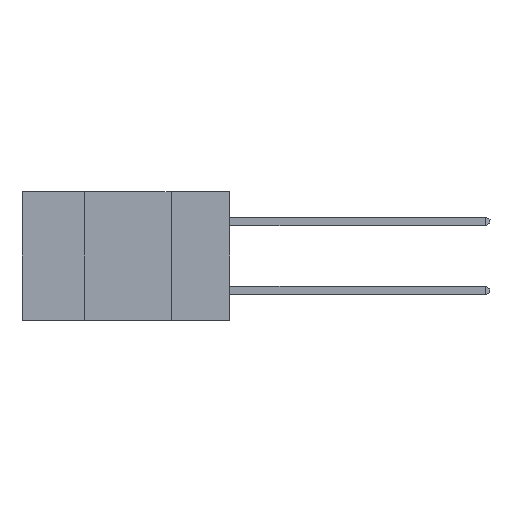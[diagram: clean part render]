
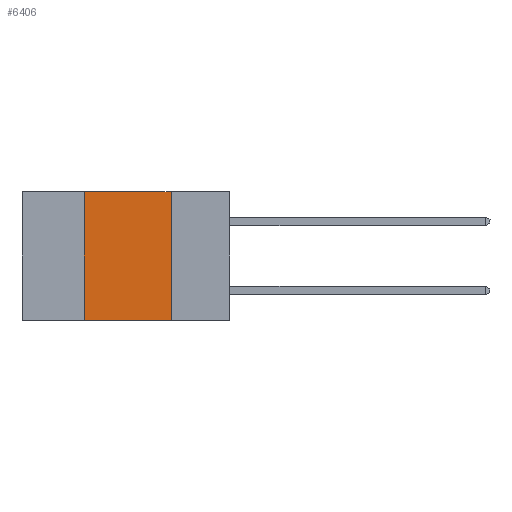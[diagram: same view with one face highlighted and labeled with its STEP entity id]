
A CAD part, left-side view. The second image highlights one B-rep face of the part: STEP entity #6406.
In plain terms, the highlighted planar face has unit normal (-1, 0, 0).
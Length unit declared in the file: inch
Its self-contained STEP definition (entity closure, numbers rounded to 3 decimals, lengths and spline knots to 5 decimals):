
#94 = FACE_OUTER_BOUND ( 'NONE', #4896, .T. ) ;
#142 = VERTEX_POINT ( 'NONE', #1710 ) ;
#200 = DIRECTION ( 'NONE',  ( 1., 0., 0. ) ) ;
#377 = VECTOR ( 'NONE', #9001, 39.37008 ) ;
#720 = CARTESIAN_POINT ( 'NONE',  ( 0., 0.42, -0.37 ) ) ;
#926 = CARTESIAN_POINT ( 'NONE',  ( 0., 0.6, 0. ) ) ;
#1450 = LINE ( 'NONE', #8286, #4616 ) ;
#1541 = DIRECTION ( 'NONE',  ( 0., 0., -1. ) ) ;
#1710 = CARTESIAN_POINT ( 'NONE',  ( 0., 0.42, 0. ) ) ;
#2389 = VERTEX_POINT ( 'NONE', #2802 ) ;
#2575 = ORIENTED_EDGE ( 'NONE', *, *, #3116, .F. ) ;
#2617 = LINE ( 'NONE', #8356, #5705 ) ;
#2663 = LINE ( 'NONE', #6421, #2665 ) ;
#2665 = VECTOR ( 'NONE', #4724, 39.37008 ) ;
#2802 = CARTESIAN_POINT ( 'NONE',  ( 0., 0.17, -0.37 ) ) ;
#3026 = CARTESIAN_POINT ( 'NONE',  ( 0., 0.17, 0. ) ) ;
#3046 = ORIENTED_EDGE ( 'NONE', *, *, #5584, .F. ) ;
#3116 = EDGE_CURVE ( 'NONE', #142, #6722, #2663, .T. ) ;
#3891 = CARTESIAN_POINT ( 'NONE',  ( 0., 0.6, -0.37 ) ) ;
#4616 = VECTOR ( 'NONE', #7342, 39.37008 ) ;
#4724 = DIRECTION ( 'NONE',  ( 0., -1., 0. ) ) ;
#4896 = EDGE_LOOP ( 'NONE', ( #3046, #2575, #5711, #8697 ) ) ;
#4983 = EDGE_CURVE ( 'NONE', #7229, #2389, #5543, .T. ) ;
#5543 = LINE ( 'NONE', #3891, #377 ) ;
#5584 = EDGE_CURVE ( 'NONE', #6722, #2389, #2617, .T. ) ;
#5705 = VECTOR ( 'NONE', #6991, 39.37008 ) ;
#5711 = ORIENTED_EDGE ( 'NONE', *, *, #6312, .F. ) ;
#6312 = EDGE_CURVE ( 'NONE', #7229, #142, #1450, .T. ) ;
#6406 = ADVANCED_FACE ( 'NONE', ( #94 ), #6910, .F. ) ;
#6421 = CARTESIAN_POINT ( 'NONE',  ( 0., 0.6, 0. ) ) ;
#6555 = AXIS2_PLACEMENT_3D ( 'NONE', #926, #200, #1541 ) ;
#6722 = VERTEX_POINT ( 'NONE', #3026 ) ;
#6910 = PLANE ( 'NONE',  #6555 ) ;
#6991 = DIRECTION ( 'NONE',  ( 0., 0., -1. ) ) ;
#7229 = VERTEX_POINT ( 'NONE', #720 ) ;
#7342 = DIRECTION ( 'NONE',  ( 0., 0., 1. ) ) ;
#8286 = CARTESIAN_POINT ( 'NONE',  ( 0., 0.42, -0.37 ) ) ;
#8356 = CARTESIAN_POINT ( 'NONE',  ( 0., 0.17, -0.37 ) ) ;
#8697 = ORIENTED_EDGE ( 'NONE', *, *, #4983, .T. ) ;
#9001 = DIRECTION ( 'NONE',  ( 0., -1., 0. ) ) ;
